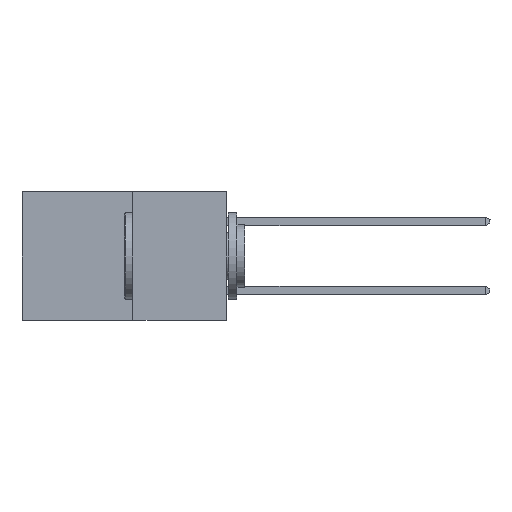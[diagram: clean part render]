
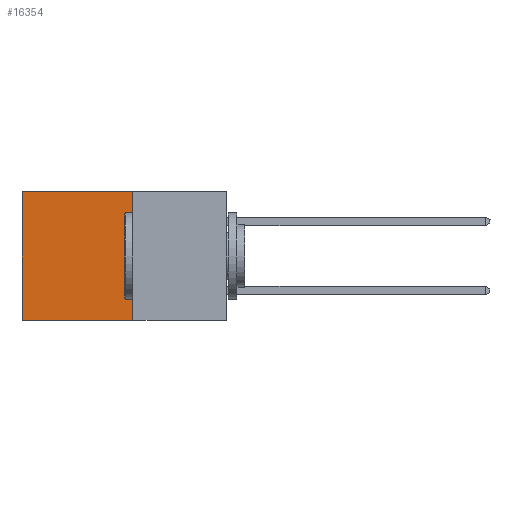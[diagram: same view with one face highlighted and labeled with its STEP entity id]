
A CAD part, left-side view. The second image highlights one B-rep face of the part: STEP entity #16354.
In plain terms, the highlighted planar face has unit normal (-1, 0, 0).
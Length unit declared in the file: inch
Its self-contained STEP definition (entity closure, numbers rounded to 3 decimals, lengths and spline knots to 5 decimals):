
#536 = DIRECTION ( 'NONE',  ( 0., 1., 0. ) ) ;
#628 = LINE ( 'NONE', #18009, #15227 ) ;
#1008 = CARTESIAN_POINT ( 'NONE',  ( 0.277, 0.59, -0.37 ) ) ;
#1191 = CARTESIAN_POINT ( 'NONE',  ( 0.277, 0.59, -0.37 ) ) ;
#2194 = DIRECTION ( 'NONE',  ( 0., 0., -1. ) ) ;
#2812 = VECTOR ( 'NONE', #10443, 39.37008 ) ;
#4059 = VERTEX_POINT ( 'NONE', #12545 ) ;
#4601 = EDGE_CURVE ( 'NONE', #22618, #6678, #628, .T. ) ;
#6298 = CARTESIAN_POINT ( 'NONE',  ( 0.277, 0.27, 0. ) ) ;
#6398 = ORIENTED_EDGE ( 'NONE', *, *, #14470, .F. ) ;
#6678 = VERTEX_POINT ( 'NONE', #7367 ) ;
#7367 = CARTESIAN_POINT ( 'NONE',  ( 0.277, 0.27, -0.37 ) ) ;
#7856 = AXIS2_PLACEMENT_3D ( 'NONE', #9861, #13627, #2194 ) ;
#8416 = ORIENTED_EDGE ( 'NONE', *, *, #13830, .T. ) ;
#8452 = VECTOR ( 'NONE', #8767, 39.37008 ) ;
#8520 = CARTESIAN_POINT ( 'NONE',  ( 0.277, 0.27, -0.37 ) ) ;
#8767 = DIRECTION ( 'NONE',  ( 0., 0., -1. ) ) ;
#9734 = ORIENTED_EDGE ( 'NONE', *, *, #16628, .T. ) ;
#9861 = CARTESIAN_POINT ( 'NONE',  ( 0.277, 0.27, -0.37 ) ) ;
#10073 = LINE ( 'NONE', #6298, #24184 ) ;
#10443 = DIRECTION ( 'NONE',  ( 0., 1., 0. ) ) ;
#12545 = CARTESIAN_POINT ( 'NONE',  ( 0.277, 0.59, 0. ) ) ;
#12984 = LINE ( 'NONE', #8520, #2812 ) ;
#13627 = DIRECTION ( 'NONE',  ( 1., 0., 0. ) ) ;
#13830 = EDGE_CURVE ( 'NONE', #22618, #4059, #10073, .T. ) ;
#14352 = CARTESIAN_POINT ( 'NONE',  ( 0.277, 0.27, 0. ) ) ;
#14470 = EDGE_CURVE ( 'NONE', #6678, #16663, #12984, .T. ) ;
#14923 = FACE_OUTER_BOUND ( 'NONE', #21844, .T. ) ;
#15227 = VECTOR ( 'NONE', #17688, 39.37008 ) ;
#16354 = ADVANCED_FACE ( 'NONE', ( #14923 ), #20938, .F. ) ;
#16628 = EDGE_CURVE ( 'NONE', #4059, #16663, #23226, .T. ) ;
#16663 = VERTEX_POINT ( 'NONE', #1191 ) ;
#17688 = DIRECTION ( 'NONE',  ( 0., 0., -1. ) ) ;
#18009 = CARTESIAN_POINT ( 'NONE',  ( 0.277, 0.27, -0.37 ) ) ;
#20938 = PLANE ( 'NONE',  #7856 ) ;
#21844 = EDGE_LOOP ( 'NONE', ( #9734, #6398, #24054, #8416 ) ) ;
#22618 = VERTEX_POINT ( 'NONE', #14352 ) ;
#23226 = LINE ( 'NONE', #1008, #8452 ) ;
#24054 = ORIENTED_EDGE ( 'NONE', *, *, #4601, .F. ) ;
#24184 = VECTOR ( 'NONE', #536, 39.37008 ) ;
